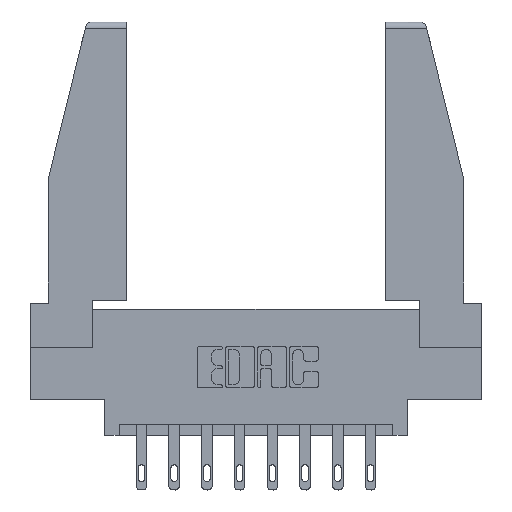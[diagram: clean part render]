
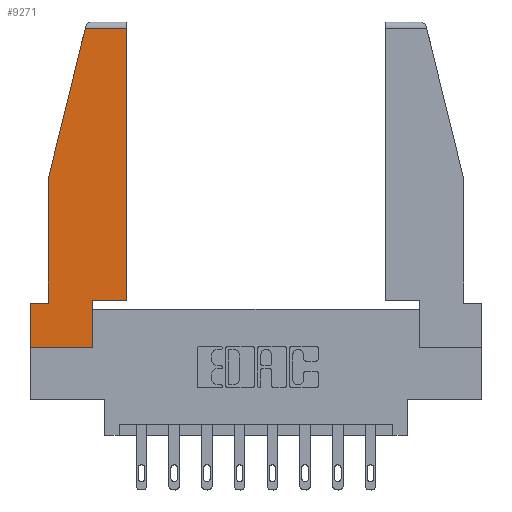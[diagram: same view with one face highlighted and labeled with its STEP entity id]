
A CAD part, top view. The second image highlights one B-rep face of the part: STEP entity #9271.
In plain terms, the highlighted planar face has unit normal (0, 0, 1).
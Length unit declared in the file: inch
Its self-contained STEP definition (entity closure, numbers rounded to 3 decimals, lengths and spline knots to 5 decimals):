
#139 = CARTESIAN_POINT ( 'NONE',  ( 0., 0.21, 0. ) ) ;
#159 = EDGE_CURVE ( 'NONE', #11758, #11367, #11841, .T. ) ;
#587 = CARTESIAN_POINT ( 'NONE',  ( 0.297, 0., 0. ) ) ;
#850 = LINE ( 'NONE', #10051, #2606 ) ;
#912 = CARTESIAN_POINT ( 'NONE',  ( 0.271, 1.55, 0. ) ) ;
#1501 = VECTOR ( 'NONE', #12644, 39.37008 ) ;
#1514 = VERTEX_POINT ( 'NONE', #6743 ) ;
#1558 = ORIENTED_EDGE ( 'NONE', *, *, #7332, .T. ) ;
#1732 = DIRECTION ( 'NONE',  ( 0., 1., 0. ) ) ;
#1818 = LINE ( 'NONE', #11800, #10704 ) ;
#1837 = DIRECTION ( 'NONE',  ( -0.239, -0.971, 0. ) ) ;
#1947 = ORIENTED_EDGE ( 'NONE', *, *, #5112, .T. ) ;
#2032 = DIRECTION ( 'NONE',  ( 0., -1., 0. ) ) ;
#2444 = VERTEX_POINT ( 'NONE', #6382 ) ;
#2487 = LINE ( 'NONE', #3763, #8812 ) ;
#2606 = VECTOR ( 'NONE', #2032, 39.37008 ) ;
#2888 = DIRECTION ( 'NONE',  ( -1., 0., 0. ) ) ;
#2948 = ORIENTED_EDGE ( 'NONE', *, *, #7124, .T. ) ;
#2962 = ORIENTED_EDGE ( 'NONE', *, *, #12594, .T. ) ;
#3242 = LINE ( 'NONE', #10526, #1501 ) ;
#3309 = VERTEX_POINT ( 'NONE', #9207 ) ;
#3646 = ORIENTED_EDGE ( 'NONE', *, *, #8682, .T. ) ;
#3647 = VERTEX_POINT ( 'NONE', #9444 ) ;
#3763 = CARTESIAN_POINT ( 'NONE',  ( 0., 0.21, 0. ) ) ;
#3773 = PLANE ( 'NONE',  #8107 ) ;
#3868 = CARTESIAN_POINT ( 'NONE',  ( 0., 1.52, 0. ) ) ;
#3908 = CARTESIAN_POINT ( 'NONE',  ( 0.297, 0., 0. ) ) ;
#3980 = DIRECTION ( 'NONE',  ( 0., -1., 0. ) ) ;
#4080 = VECTOR ( 'NONE', #11459, 39.37008 ) ;
#4293 = FACE_OUTER_BOUND ( 'NONE', #10502, .T. ) ;
#4557 = VERTEX_POINT ( 'NONE', #5213 ) ;
#4718 = CARTESIAN_POINT ( 'NONE',  ( 0.086, 0.21, 0. ) ) ;
#4993 = CARTESIAN_POINT ( 'NONE',  ( 0., 0.21, 0. ) ) ;
#5112 = EDGE_CURVE ( 'NONE', #3309, #3647, #7574, .T. ) ;
#5213 = CARTESIAN_POINT ( 'NONE',  ( 0.461, 0.223, 0. ) ) ;
#5401 = VECTOR ( 'NONE', #11093, 39.37008 ) ;
#5489 = LINE ( 'NONE', #3868, #8204 ) ;
#5606 = ORIENTED_EDGE ( 'NONE', *, *, #7459, .T. ) ;
#5616 = VECTOR ( 'NONE', #12099, 39.37008 ) ;
#5811 = EDGE_CURVE ( 'NONE', #7754, #3309, #5489, .T. ) ;
#6382 = CARTESIAN_POINT ( 'NONE',  ( 0.297, 0.223, 0. ) ) ;
#6743 = CARTESIAN_POINT ( 'NONE',  ( 0., 0., 0. ) ) ;
#6780 = VECTOR ( 'NONE', #1837, 39.37008 ) ;
#7007 = CARTESIAN_POINT ( 'NONE',  ( 0., 0., 0. ) ) ;
#7124 = EDGE_CURVE ( 'NONE', #4557, #7754, #1818, .T. ) ;
#7332 = EDGE_CURVE ( 'NONE', #3647, #11758, #850, .T. ) ;
#7459 = EDGE_CURVE ( 'NONE', #2444, #4557, #3242, .T. ) ;
#7574 = LINE ( 'NONE', #912, #6780 ) ;
#7754 = VERTEX_POINT ( 'NONE', #12604 ) ;
#8107 = AXIS2_PLACEMENT_3D ( 'NONE', #7007, #13065, #9974 ) ;
#8204 = VECTOR ( 'NONE', #2888, 39.37008 ) ;
#8268 = LINE ( 'NONE', #3908, #5401 ) ;
#8682 = EDGE_CURVE ( 'NONE', #12528, #2444, #8268, .T. ) ;
#8812 = VECTOR ( 'NONE', #3980, 39.37008 ) ;
#9207 = CARTESIAN_POINT ( 'NONE',  ( 0.2636, 1.52, 0. ) ) ;
#9208 = CARTESIAN_POINT ( 'NONE',  ( 0., 0., 0. ) ) ;
#9271 = ADVANCED_FACE ( 'NONE', ( #4293 ), #3773, .T. ) ;
#9444 = CARTESIAN_POINT ( 'NONE',  ( 0.086, 0.8, 0. ) ) ;
#9974 = DIRECTION ( 'NONE',  ( 1., 0., 0. ) ) ;
#10051 = CARTESIAN_POINT ( 'NONE',  ( 0.086, 0.8, 0. ) ) ;
#10267 = ORIENTED_EDGE ( 'NONE', *, *, #5811, .T. ) ;
#10502 = EDGE_LOOP ( 'NONE', ( #2948, #10267, #1947, #1558, #11784, #2962, #11601, #3646, #5606 ) ) ;
#10526 = CARTESIAN_POINT ( 'NONE',  ( 0.297, 0.223, 0. ) ) ;
#10704 = VECTOR ( 'NONE', #1732, 39.37008 ) ;
#11093 = DIRECTION ( 'NONE',  ( 0., 1., 0. ) ) ;
#11367 = VERTEX_POINT ( 'NONE', #139 ) ;
#11459 = DIRECTION ( 'NONE',  ( 1., 0., 0. ) ) ;
#11601 = ORIENTED_EDGE ( 'NONE', *, *, #12294, .T. ) ;
#11758 = VERTEX_POINT ( 'NONE', #4718 ) ;
#11784 = ORIENTED_EDGE ( 'NONE', *, *, #159, .T. ) ;
#11800 = CARTESIAN_POINT ( 'NONE',  ( 0.461, 0.223, 0. ) ) ;
#11841 = LINE ( 'NONE', #4993, #5616 ) ;
#12099 = DIRECTION ( 'NONE',  ( -1., 0., 0. ) ) ;
#12294 = EDGE_CURVE ( 'NONE', #1514, #12528, #12944, .T. ) ;
#12528 = VERTEX_POINT ( 'NONE', #587 ) ;
#12594 = EDGE_CURVE ( 'NONE', #11367, #1514, #2487, .T. ) ;
#12604 = CARTESIAN_POINT ( 'NONE',  ( 0.461, 1.52, 0. ) ) ;
#12644 = DIRECTION ( 'NONE',  ( 1., 0., 0. ) ) ;
#12944 = LINE ( 'NONE', #9208, #4080 ) ;
#13065 = DIRECTION ( 'NONE',  ( 0., 0., 1. ) ) ;
